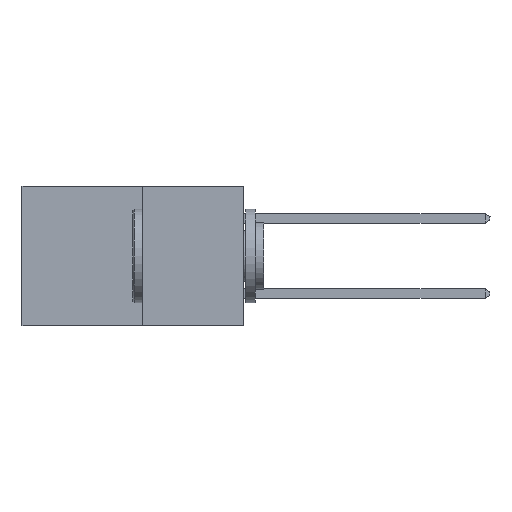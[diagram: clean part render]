
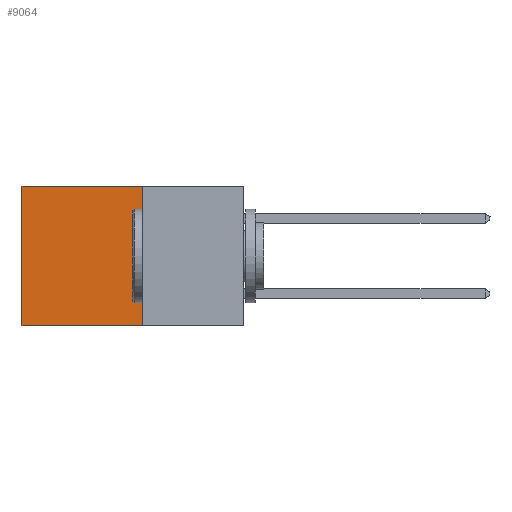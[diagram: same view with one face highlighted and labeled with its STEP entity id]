
A CAD part, left-side view. The second image highlights one B-rep face of the part: STEP entity #9064.
In plain terms, the highlighted planar face has unit normal (-1, 0, 0).
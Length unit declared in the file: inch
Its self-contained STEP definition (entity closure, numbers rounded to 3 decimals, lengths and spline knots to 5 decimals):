
#252 = DIRECTION ( 'NONE',  ( 0., 1., 0. ) ) ;
#308 = VERTEX_POINT ( 'NONE', #6427 ) ;
#517 = LINE ( 'NONE', #14061, #16499 ) ;
#1149 = LINE ( 'NONE', #10153, #8307 ) ;
#1638 = CARTESIAN_POINT ( 'NONE',  ( 0.277, 0.27, 0. ) ) ;
#1703 = CARTESIAN_POINT ( 'NONE',  ( 0.277, 0.27, -0.37 ) ) ;
#3378 = PLANE ( 'NONE',  #8532 ) ;
#4920 = ORIENTED_EDGE ( 'NONE', *, *, #10187, .F. ) ;
#5354 = ORIENTED_EDGE ( 'NONE', *, *, #9036, .T. ) ;
#6291 = DIRECTION ( 'NONE',  ( 0., 0., -1. ) ) ;
#6427 = CARTESIAN_POINT ( 'NONE',  ( 0.277, 0.59, -0.37 ) ) ;
#7975 = VECTOR ( 'NONE', #12892, 39.37008 ) ;
#8307 = VECTOR ( 'NONE', #252, 39.37008 ) ;
#8532 = AXIS2_PLACEMENT_3D ( 'NONE', #1703, #14725, #6291 ) ;
#8965 = LINE ( 'NONE', #9979, #16047 ) ;
#9036 = EDGE_CURVE ( 'NONE', #12284, #12502, #11200, .T. ) ;
#9064 = ADVANCED_FACE ( 'NONE', ( #10282 ), #3378, .F. ) ;
#9776 = CARTESIAN_POINT ( 'NONE',  ( 0.277, 0.59, 0. ) ) ;
#9979 = CARTESIAN_POINT ( 'NONE',  ( 0.277, 0.59, -0.37 ) ) ;
#10153 = CARTESIAN_POINT ( 'NONE',  ( 0.277, 0.27, -0.37 ) ) ;
#10187 = EDGE_CURVE ( 'NONE', #12284, #14585, #517, .T. ) ;
#10282 = FACE_OUTER_BOUND ( 'NONE', #15584, .T. ) ;
#10516 = ORIENTED_EDGE ( 'NONE', *, *, #15900, .T. ) ;
#10901 = CARTESIAN_POINT ( 'NONE',  ( 0.277, 0.27, -0.37 ) ) ;
#11200 = LINE ( 'NONE', #1638, #7975 ) ;
#11432 = DIRECTION ( 'NONE',  ( 0., 0., -1. ) ) ;
#11435 = ORIENTED_EDGE ( 'NONE', *, *, #11973, .F. ) ;
#11973 = EDGE_CURVE ( 'NONE', #14585, #308, #1149, .T. ) ;
#12284 = VERTEX_POINT ( 'NONE', #13661 ) ;
#12502 = VERTEX_POINT ( 'NONE', #9776 ) ;
#12892 = DIRECTION ( 'NONE',  ( 0., 1., 0. ) ) ;
#13661 = CARTESIAN_POINT ( 'NONE',  ( 0.277, 0.27, 0. ) ) ;
#13992 = DIRECTION ( 'NONE',  ( 0., 0., -1. ) ) ;
#14061 = CARTESIAN_POINT ( 'NONE',  ( 0.277, 0.27, -0.37 ) ) ;
#14585 = VERTEX_POINT ( 'NONE', #10901 ) ;
#14725 = DIRECTION ( 'NONE',  ( 1., 0., 0. ) ) ;
#15584 = EDGE_LOOP ( 'NONE', ( #10516, #11435, #4920, #5354 ) ) ;
#15900 = EDGE_CURVE ( 'NONE', #12502, #308, #8965, .T. ) ;
#16047 = VECTOR ( 'NONE', #11432, 39.37008 ) ;
#16499 = VECTOR ( 'NONE', #13992, 39.37008 ) ;
